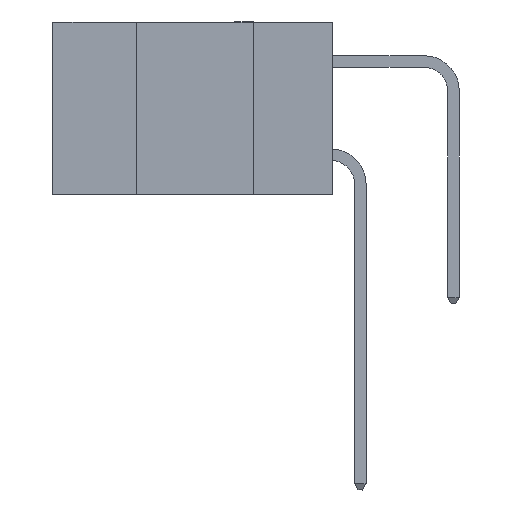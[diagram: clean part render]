
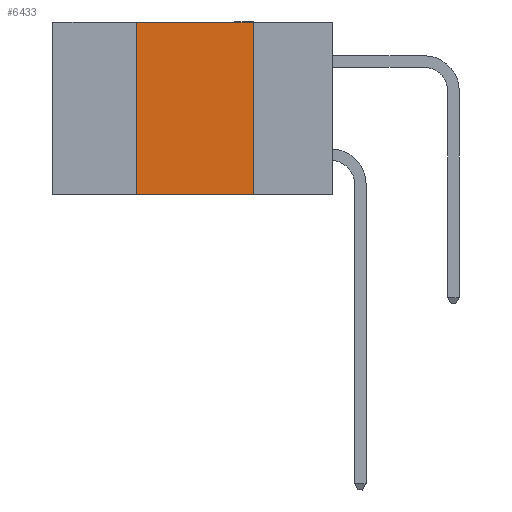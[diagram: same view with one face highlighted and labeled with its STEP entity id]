
A CAD part, left-side view. The second image highlights one B-rep face of the part: STEP entity #6433.
In plain terms, the highlighted planar face has unit normal (-1, 0, 0).
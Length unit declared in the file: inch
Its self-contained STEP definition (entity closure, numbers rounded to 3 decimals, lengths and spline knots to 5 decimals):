
#223 = FACE_OUTER_BOUND ( 'NONE', #13224, .T. ) ;
#616 = EDGE_CURVE ( 'NONE', #10081, #5041, #12166, .T. ) ;
#1821 = VERTEX_POINT ( 'NONE', #2520 ) ;
#2171 = DIRECTION ( 'NONE',  ( 0., 0., -1. ) ) ;
#2520 = CARTESIAN_POINT ( 'NONE',  ( 0., 0.17, -0.37 ) ) ;
#3724 = EDGE_CURVE ( 'NONE', #5041, #15760, #8636, .T. ) ;
#3957 = EDGE_CURVE ( 'NONE', #10081, #1821, #11438, .T. ) ;
#4582 = CARTESIAN_POINT ( 'NONE',  ( 0., 0.17, 0. ) ) ;
#5041 = VERTEX_POINT ( 'NONE', #11792 ) ;
#5463 = LINE ( 'NONE', #4582, #14456 ) ;
#5720 = ORIENTED_EDGE ( 'NONE', *, *, #616, .F. ) ;
#5948 = VECTOR ( 'NONE', #11028, 39.37008 ) ;
#5951 = CARTESIAN_POINT ( 'NONE',  ( 0., 0.6, -0.37 ) ) ;
#6038 = DIRECTION ( 'NONE',  ( 0., 0., -1. ) ) ;
#6103 = CARTESIAN_POINT ( 'NONE',  ( 0., 0.17, 0. ) ) ;
#6433 = ADVANCED_FACE ( 'NONE', ( #223 ), #12364, .F. ) ;
#6466 = VECTOR ( 'NONE', #7827, 39.37008 ) ;
#6548 = CARTESIAN_POINT ( 'NONE',  ( 0., 0.6, 0. ) ) ;
#6845 = ORIENTED_EDGE ( 'NONE', *, *, #13335, .F. ) ;
#7827 = DIRECTION ( 'NONE',  ( 0., -1., 0. ) ) ;
#8560 = DIRECTION ( 'NONE',  ( 1., 0., 0. ) ) ;
#8628 = ORIENTED_EDGE ( 'NONE', *, *, #3957, .T. ) ;
#8636 = LINE ( 'NONE', #6548, #6466 ) ;
#9844 = CARTESIAN_POINT ( 'NONE',  ( 0., 0.6, 0. ) ) ;
#9879 = ORIENTED_EDGE ( 'NONE', *, *, #3724, .F. ) ;
#10081 = VERTEX_POINT ( 'NONE', #10779 ) ;
#10779 = CARTESIAN_POINT ( 'NONE',  ( 0., 0.42, -0.37 ) ) ;
#11028 = DIRECTION ( 'NONE',  ( 0., 0., 1. ) ) ;
#11438 = LINE ( 'NONE', #5951, #15404 ) ;
#11792 = CARTESIAN_POINT ( 'NONE',  ( 0., 0.42, 0. ) ) ;
#12166 = LINE ( 'NONE', #15004, #5948 ) ;
#12364 = PLANE ( 'NONE',  #13947 ) ;
#13224 = EDGE_LOOP ( 'NONE', ( #6845, #9879, #5720, #8628 ) ) ;
#13335 = EDGE_CURVE ( 'NONE', #15760, #1821, #5463, .T. ) ;
#13947 = AXIS2_PLACEMENT_3D ( 'NONE', #9844, #8560, #6038 ) ;
#14456 = VECTOR ( 'NONE', #2171, 39.37008 ) ;
#14861 = DIRECTION ( 'NONE',  ( 0., -1., 0. ) ) ;
#15004 = CARTESIAN_POINT ( 'NONE',  ( 0., 0.42, 0. ) ) ;
#15404 = VECTOR ( 'NONE', #14861, 39.37008 ) ;
#15760 = VERTEX_POINT ( 'NONE', #6103 ) ;
